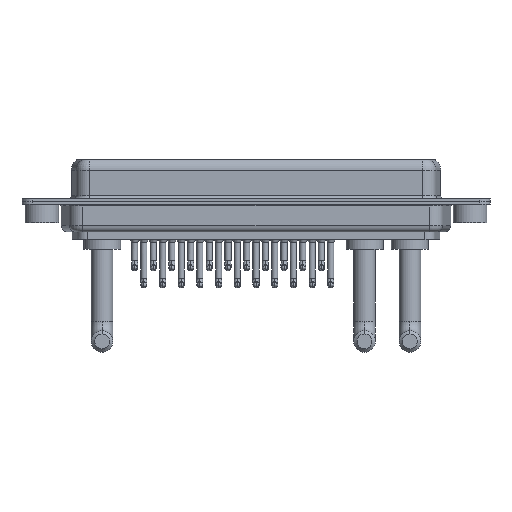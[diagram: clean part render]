
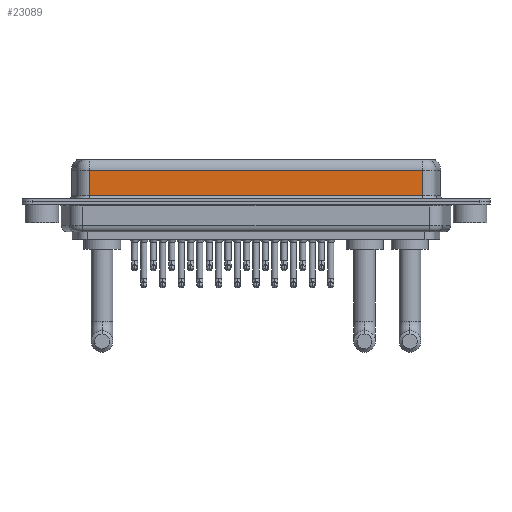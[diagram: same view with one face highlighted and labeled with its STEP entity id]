
A CAD part, front view. The second image highlights one B-rep face of the part: STEP entity #23089.
In plain terms, the highlighted planar face has unit normal (0, -1, 0).
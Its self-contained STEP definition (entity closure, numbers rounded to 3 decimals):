
#669 = VECTOR ( 'NONE', #22681, 1000. ) ;
#2164 = CARTESIAN_POINT ( 'NONE',  ( 56.462, -3.95, 6.4 ) ) ;
#2774 = DIRECTION ( 'NONE',  ( 1., 0., 0. ) ) ;
#3065 = EDGE_CURVE ( 'NONE', #21351, #13056, #6445, .T. ) ;
#3407 = CARTESIAN_POINT ( 'NONE',  ( 7.038, -3.95, 4.65 ) ) ;
#4336 = DIRECTION ( 'NONE',  ( 0., 0., -1. ) ) ;
#5389 = ORIENTED_EDGE ( 'NONE', *, *, #13038, .F. ) ;
#5615 = VECTOR ( 'NONE', #2774, 1000. ) ;
#5666 = PLANE ( 'NONE',  #11409 ) ;
#5698 = VECTOR ( 'NONE', #4336, 1000. ) ;
#6445 = LINE ( 'NONE', #20989, #669 ) ;
#6787 = VECTOR ( 'NONE', #23550, 1000. ) ;
#8936 = ORIENTED_EDGE ( 'NONE', *, *, #22769, .T. ) ;
#9666 = DIRECTION ( 'NONE',  ( 0., 1., 0. ) ) ;
#10496 = ORIENTED_EDGE ( 'NONE', *, *, #3065, .T. ) ;
#11195 = CARTESIAN_POINT ( 'NONE',  ( 56.462, -3.95, 0.9 ) ) ;
#11409 = AXIS2_PLACEMENT_3D ( 'NONE', #2164, #9666, #18811 ) ;
#11930 = LINE ( 'NONE', #15945, #5698 ) ;
#12111 = CARTESIAN_POINT ( 'NONE',  ( 56.462, -3.95, 6.4 ) ) ;
#12222 = LINE ( 'NONE', #12111, #6787 ) ;
#13038 = EDGE_CURVE ( 'NONE', #21351, #22177, #12222, .T. ) ;
#13056 = VERTEX_POINT ( 'NONE', #3407 ) ;
#13330 = EDGE_CURVE ( 'NONE', #13056, #13875, #11930, .T. ) ;
#13875 = VERTEX_POINT ( 'NONE', #23583 ) ;
#14640 = ORIENTED_EDGE ( 'NONE', *, *, #13330, .T. ) ;
#15945 = CARTESIAN_POINT ( 'NONE',  ( 7.038, -3.95, 6.4 ) ) ;
#18446 = EDGE_LOOP ( 'NONE', ( #5389, #10496, #14640, #8936 ) ) ;
#18695 = FACE_OUTER_BOUND ( 'NONE', #18446, .T. ) ;
#18811 = DIRECTION ( 'NONE',  ( 0., 0., 1. ) ) ;
#19323 = CARTESIAN_POINT ( 'NONE',  ( 56.462, -3.95, 0.9 ) ) ;
#20660 = CARTESIAN_POINT ( 'NONE',  ( 56.462, -3.95, 4.65 ) ) ;
#20989 = CARTESIAN_POINT ( 'NONE',  ( 56.462, -3.95, 4.65 ) ) ;
#21351 = VERTEX_POINT ( 'NONE', #20660 ) ;
#22177 = VERTEX_POINT ( 'NONE', #11195 ) ;
#22681 = DIRECTION ( 'NONE',  ( -1., 0., 0. ) ) ;
#22769 = EDGE_CURVE ( 'NONE', #13875, #22177, #22940, .T. ) ;
#22940 = LINE ( 'NONE', #19323, #5615 ) ;
#23089 = ADVANCED_FACE ( 'NONE', ( #18695 ), #5666, .F. ) ;
#23550 = DIRECTION ( 'NONE',  ( 0., 0., -1. ) ) ;
#23583 = CARTESIAN_POINT ( 'NONE',  ( 7.038, -3.95, 0.9 ) ) ;
